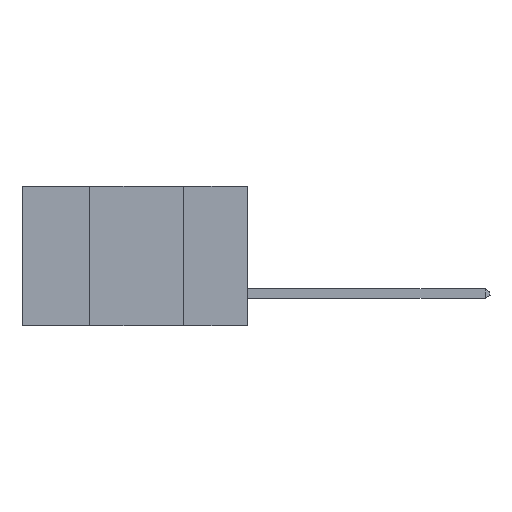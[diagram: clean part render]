
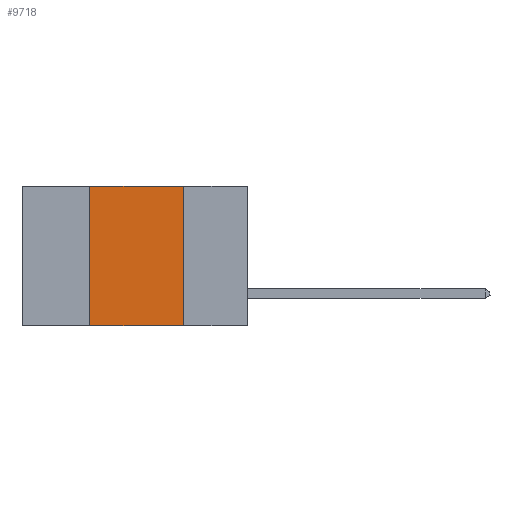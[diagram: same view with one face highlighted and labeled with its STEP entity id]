
A CAD part, left-side view. The second image highlights one B-rep face of the part: STEP entity #9718.
In plain terms, the highlighted planar face has unit normal (-1, 0, 0).
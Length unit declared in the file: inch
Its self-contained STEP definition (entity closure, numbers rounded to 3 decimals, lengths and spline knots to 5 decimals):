
#102 = VERTEX_POINT ( 'NONE', #7407 ) ;
#288 = DIRECTION ( 'NONE',  ( 0., 0., -1. ) ) ;
#663 = VECTOR ( 'NONE', #288, 39.37008 ) ;
#1017 = VERTEX_POINT ( 'NONE', #12865 ) ;
#2033 = VECTOR ( 'NONE', #5694, 39.37008 ) ;
#2133 = CARTESIAN_POINT ( 'NONE',  ( 0., 0.42, 0. ) ) ;
#2634 = VECTOR ( 'NONE', #11917, 39.37008 ) ;
#2709 = LINE ( 'NONE', #2133, #7205 ) ;
#2913 = CARTESIAN_POINT ( 'NONE',  ( 0., 0.42, 0. ) ) ;
#2943 = LINE ( 'NONE', #10802, #2634 ) ;
#3137 = VERTEX_POINT ( 'NONE', #4010 ) ;
#3562 = ORIENTED_EDGE ( 'NONE', *, *, #7155, .T. ) ;
#4010 = CARTESIAN_POINT ( 'NONE',  ( 0., 0.42, -0.37 ) ) ;
#5304 = PLANE ( 'NONE',  #9604 ) ;
#5500 = EDGE_LOOP ( 'NONE', ( #6912, #12249, #5927, #3562 ) ) ;
#5645 = EDGE_CURVE ( 'NONE', #11859, #102, #10418, .T. ) ;
#5694 = DIRECTION ( 'NONE',  ( 0., -1., 0. ) ) ;
#5927 = ORIENTED_EDGE ( 'NONE', *, *, #9696, .F. ) ;
#6203 = DIRECTION ( 'NONE',  ( 0., 0., -1. ) ) ;
#6912 = ORIENTED_EDGE ( 'NONE', *, *, #12890, .F. ) ;
#7155 = EDGE_CURVE ( 'NONE', #3137, #1017, #2943, .T. ) ;
#7205 = VECTOR ( 'NONE', #11066, 39.37008 ) ;
#7407 = CARTESIAN_POINT ( 'NONE',  ( 0., 0.17, 0. ) ) ;
#7668 = FACE_OUTER_BOUND ( 'NONE', #5500, .T. ) ;
#8313 = DIRECTION ( 'NONE',  ( 1., 0., 0. ) ) ;
#9353 = CARTESIAN_POINT ( 'NONE',  ( 0., 0.17, 0. ) ) ;
#9604 = AXIS2_PLACEMENT_3D ( 'NONE', #10258, #8313, #6203 ) ;
#9696 = EDGE_CURVE ( 'NONE', #3137, #11859, #2709, .T. ) ;
#9718 = ADVANCED_FACE ( 'NONE', ( #7668 ), #5304, .F. ) ;
#10258 = CARTESIAN_POINT ( 'NONE',  ( 0., 0.6, 0. ) ) ;
#10418 = LINE ( 'NONE', #12728, #2033 ) ;
#10802 = CARTESIAN_POINT ( 'NONE',  ( 0., 0.6, -0.37 ) ) ;
#11066 = DIRECTION ( 'NONE',  ( 0., 0., 1. ) ) ;
#11084 = LINE ( 'NONE', #9353, #663 ) ;
#11859 = VERTEX_POINT ( 'NONE', #2913 ) ;
#11917 = DIRECTION ( 'NONE',  ( 0., -1., 0. ) ) ;
#12249 = ORIENTED_EDGE ( 'NONE', *, *, #5645, .F. ) ;
#12728 = CARTESIAN_POINT ( 'NONE',  ( 0., 0.6, 0. ) ) ;
#12865 = CARTESIAN_POINT ( 'NONE',  ( 0., 0.17, -0.37 ) ) ;
#12890 = EDGE_CURVE ( 'NONE', #102, #1017, #11084, .T. ) ;
